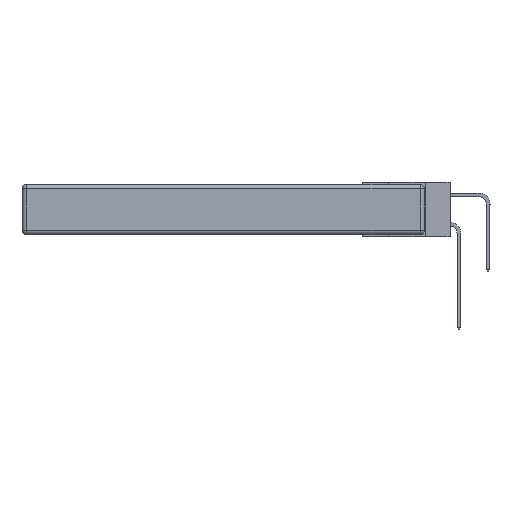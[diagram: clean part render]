
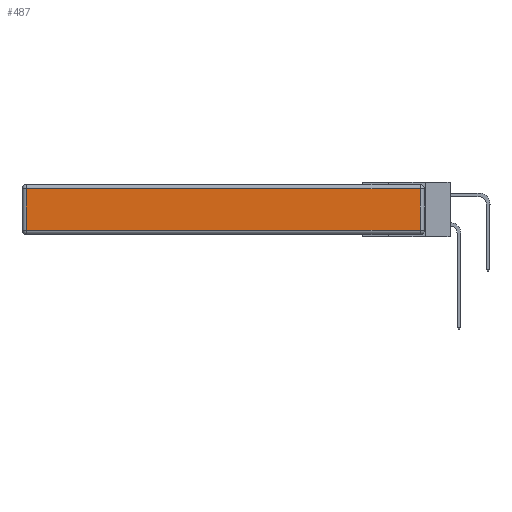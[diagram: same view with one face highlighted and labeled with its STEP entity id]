
A CAD part, left-side view. The second image highlights one B-rep face of the part: STEP entity #487.
In plain terms, the highlighted planar face has unit normal (-1, 0, 0).
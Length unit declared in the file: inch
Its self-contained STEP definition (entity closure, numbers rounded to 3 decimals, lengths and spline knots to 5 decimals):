
#487 = ADVANCED_FACE ( 'NONE', ( #12674 ), #13385, .T. ) ;
#1253 = CARTESIAN_POINT ( 'NONE',  ( 0., 0.03, -0.313 ) ) ;
#1652 = DIRECTION ( 'NONE',  ( 0., 1., 0. ) ) ;
#2276 = VECTOR ( 'NONE', #4267, 39.37008 ) ;
#2625 = EDGE_LOOP ( 'NONE', ( #4562, #10374, #12552, #7843 ) ) ;
#2747 = DIRECTION ( 'NONE',  ( 0., -1., 0. ) ) ;
#3068 = CARTESIAN_POINT ( 'NONE',  ( 0., 0., -0.343 ) ) ;
#3130 = DIRECTION ( 'NONE',  ( 0., 0., 1. ) ) ;
#3436 = VECTOR ( 'NONE', #2747, 39.37008 ) ;
#3841 = CARTESIAN_POINT ( 'NONE',  ( 0., 0., -0.313 ) ) ;
#4040 = LINE ( 'NONE', #3841, #3436 ) ;
#4267 = DIRECTION ( 'NONE',  ( 0., 0., 1. ) ) ;
#4562 = ORIENTED_EDGE ( 'NONE', *, *, #13160, .T. ) ;
#5250 = DIRECTION ( 'NONE',  ( 0., 0., -1. ) ) ;
#5306 = CARTESIAN_POINT ( 'NONE',  ( 0., 2.72, -0.343 ) ) ;
#5512 = EDGE_CURVE ( 'NONE', #16563, #6963, #11761, .T. ) ;
#5866 = VECTOR ( 'NONE', #1652, 39.37008 ) ;
#6963 = VERTEX_POINT ( 'NONE', #9062 ) ;
#7547 = VERTEX_POINT ( 'NONE', #10310 ) ;
#7643 = EDGE_CURVE ( 'NONE', #7547, #16563, #9911, .T. ) ;
#7843 = ORIENTED_EDGE ( 'NONE', *, *, #5512, .T. ) ;
#7928 = EDGE_CURVE ( 'NONE', #14221, #7547, #9495, .T. ) ;
#7944 = AXIS2_PLACEMENT_3D ( 'NONE', #3068, #15790, #3130 ) ;
#8301 = VECTOR ( 'NONE', #5250, 39.37008 ) ;
#9062 = CARTESIAN_POINT ( 'NONE',  ( 0., 2.72, -0.313 ) ) ;
#9376 = CARTESIAN_POINT ( 'NONE',  ( 0., 2.75, -0.03 ) ) ;
#9495 = LINE ( 'NONE', #12070, #2276 ) ;
#9911 = LINE ( 'NONE', #9376, #5866 ) ;
#10310 = CARTESIAN_POINT ( 'NONE',  ( 0., 0.03, -0.03 ) ) ;
#10374 = ORIENTED_EDGE ( 'NONE', *, *, #7928, .T. ) ;
#11761 = LINE ( 'NONE', #5306, #8301 ) ;
#12070 = CARTESIAN_POINT ( 'NONE',  ( 0., 0.03, -0.343 ) ) ;
#12364 = CARTESIAN_POINT ( 'NONE',  ( 0., 2.72, -0.03 ) ) ;
#12552 = ORIENTED_EDGE ( 'NONE', *, *, #7643, .T. ) ;
#12674 = FACE_OUTER_BOUND ( 'NONE', #2625, .T. ) ;
#13160 = EDGE_CURVE ( 'NONE', #6963, #14221, #4040, .T. ) ;
#13385 = PLANE ( 'NONE',  #7944 ) ;
#14221 = VERTEX_POINT ( 'NONE', #1253 ) ;
#15790 = DIRECTION ( 'NONE',  ( -1., 0., 0. ) ) ;
#16563 = VERTEX_POINT ( 'NONE', #12364 ) ;
